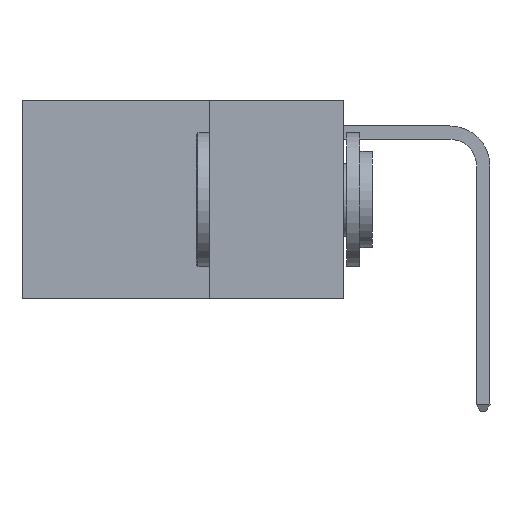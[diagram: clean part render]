
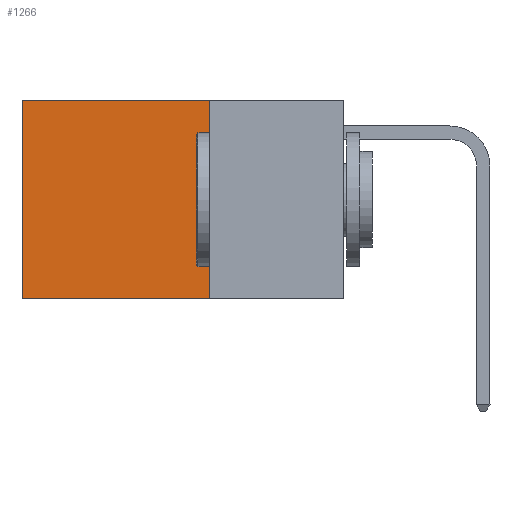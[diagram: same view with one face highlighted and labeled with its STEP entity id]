
A CAD part, left-side view. The second image highlights one B-rep face of the part: STEP entity #1266.
In plain terms, the highlighted planar face has unit normal (-1, 0, 0).
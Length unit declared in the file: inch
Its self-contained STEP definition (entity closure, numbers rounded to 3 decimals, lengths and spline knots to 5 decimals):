
#6 = VERTEX_POINT ( 'NONE', #15833 ) ;
#547 = VECTOR ( 'NONE', #3269, 39.37008 ) ;
#1266 = ADVANCED_FACE ( 'NONE', ( #8195 ), #12431, .F. ) ;
#1747 = CARTESIAN_POINT ( 'NONE',  ( 0.2625, 0.25, 0. ) ) ;
#2931 = CARTESIAN_POINT ( 'NONE',  ( 0.2625, 0.25, 0. ) ) ;
#3053 = DIRECTION ( 'NONE',  ( 0., 0., -1. ) ) ;
#3269 = DIRECTION ( 'NONE',  ( 0., 0., -1. ) ) ;
#3452 = DIRECTION ( 'NONE',  ( 0., 1., 0. ) ) ;
#4343 = VECTOR ( 'NONE', #3452, 39.37008 ) ;
#4344 = EDGE_CURVE ( 'NONE', #13794, #6, #6242, .T. ) ;
#4706 = VERTEX_POINT ( 'NONE', #12506 ) ;
#4813 = CARTESIAN_POINT ( 'NONE',  ( 0.2625, 0.6, 0. ) ) ;
#5051 = VERTEX_POINT ( 'NONE', #1747 ) ;
#5078 = CARTESIAN_POINT ( 'NONE',  ( 0.2625, 0.25, -0.37 ) ) ;
#5390 = EDGE_LOOP ( 'NONE', ( #15066, #12140, #7928, #11402 ) ) ;
#5545 = CARTESIAN_POINT ( 'NONE',  ( 0.2625, 0.25, 0. ) ) ;
#6242 = LINE ( 'NONE', #11333, #15944 ) ;
#7928 = ORIENTED_EDGE ( 'NONE', *, *, #14959, .F. ) ;
#8041 = EDGE_CURVE ( 'NONE', #5051, #13794, #15923, .T. ) ;
#8195 = FACE_OUTER_BOUND ( 'NONE', #5390, .T. ) ;
#8336 = LINE ( 'NONE', #13606, #547 ) ;
#8539 = DIRECTION ( 'NONE',  ( 1., 0., 0. ) ) ;
#10304 = VECTOR ( 'NONE', #10494, 39.37008 ) ;
#10494 = DIRECTION ( 'NONE',  ( 0., 1., 0. ) ) ;
#11333 = CARTESIAN_POINT ( 'NONE',  ( 0.2625, 0.6, 0. ) ) ;
#11402 = ORIENTED_EDGE ( 'NONE', *, *, #8041, .T. ) ;
#11444 = LINE ( 'NONE', #5078, #4343 ) ;
#12140 = ORIENTED_EDGE ( 'NONE', *, *, #13320, .F. ) ;
#12431 = PLANE ( 'NONE',  #15707 ) ;
#12506 = CARTESIAN_POINT ( 'NONE',  ( 0.2625, 0.25, -0.37 ) ) ;
#13320 = EDGE_CURVE ( 'NONE', #4706, #6, #11444, .T. ) ;
#13606 = CARTESIAN_POINT ( 'NONE',  ( 0.2625, 0.25, 0. ) ) ;
#13794 = VERTEX_POINT ( 'NONE', #4813 ) ;
#14959 = EDGE_CURVE ( 'NONE', #5051, #4706, #8336, .T. ) ;
#15066 = ORIENTED_EDGE ( 'NONE', *, *, #4344, .T. ) ;
#15707 = AXIS2_PLACEMENT_3D ( 'NONE', #5545, #8539, #3053 ) ;
#15833 = CARTESIAN_POINT ( 'NONE',  ( 0.2625, 0.6, -0.37 ) ) ;
#15923 = LINE ( 'NONE', #2931, #10304 ) ;
#15944 = VECTOR ( 'NONE', #16751, 39.37008 ) ;
#16751 = DIRECTION ( 'NONE',  ( 0., 0., -1. ) ) ;
